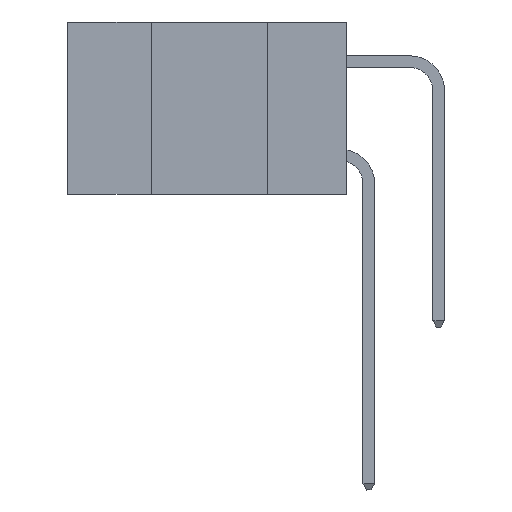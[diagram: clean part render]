
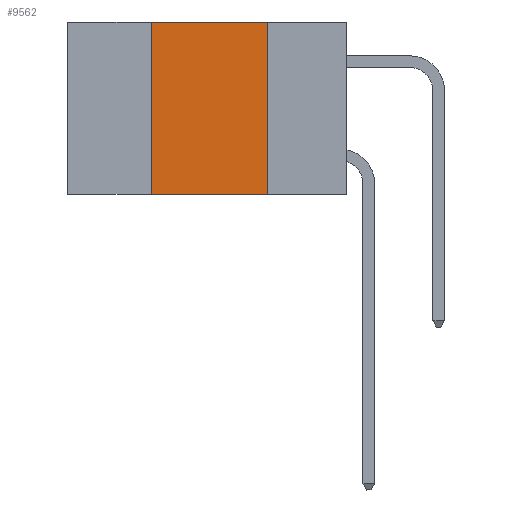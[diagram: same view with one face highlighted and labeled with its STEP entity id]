
A CAD part, left-side view. The second image highlights one B-rep face of the part: STEP entity #9562.
In plain terms, the highlighted planar face has unit normal (-1, 0, 0).
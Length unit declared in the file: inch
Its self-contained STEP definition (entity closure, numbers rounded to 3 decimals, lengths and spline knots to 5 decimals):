
#205 = DIRECTION ( 'NONE',  ( 0., -1., 0. ) ) ;
#664 = DIRECTION ( 'NONE',  ( 0., -1., 0. ) ) ;
#1040 = EDGE_CURVE ( 'NONE', #8376, #10038, #11381, .T. ) ;
#1263 = CARTESIAN_POINT ( 'NONE',  ( 0., 0.42, -0.37 ) ) ;
#1429 = ORIENTED_EDGE ( 'NONE', *, *, #1040, .F. ) ;
#1773 = LINE ( 'NONE', #12435, #2901 ) ;
#1972 = CARTESIAN_POINT ( 'NONE',  ( 0., 0.42, 0. ) ) ;
#2851 = CARTESIAN_POINT ( 'NONE',  ( 0., 0.6, 0. ) ) ;
#2901 = VECTOR ( 'NONE', #664, 39.37008 ) ;
#3010 = ORIENTED_EDGE ( 'NONE', *, *, #9655, .F. ) ;
#3097 = LINE ( 'NONE', #1972, #10056 ) ;
#3177 = DIRECTION ( 'NONE',  ( 0., 0., 1. ) ) ;
#3874 = EDGE_LOOP ( 'NONE', ( #1429, #3010, #5778, #11550 ) ) ;
#3967 = FACE_OUTER_BOUND ( 'NONE', #3874, .T. ) ;
#4256 = VERTEX_POINT ( 'NONE', #1263 ) ;
#4943 = CARTESIAN_POINT ( 'NONE',  ( 0., 0.17, 0. ) ) ;
#5388 = AXIS2_PLACEMENT_3D ( 'NONE', #2851, #13173, #6551 ) ;
#5728 = CARTESIAN_POINT ( 'NONE',  ( 0., 0.17, -0.37 ) ) ;
#5778 = ORIENTED_EDGE ( 'NONE', *, *, #14907, .F. ) ;
#6551 = DIRECTION ( 'NONE',  ( 0., 0., -1. ) ) ;
#7616 = EDGE_CURVE ( 'NONE', #4256, #10038, #1773, .T. ) ;
#8175 = CARTESIAN_POINT ( 'NONE',  ( 0., 0.17, 0. ) ) ;
#8376 = VERTEX_POINT ( 'NONE', #8175 ) ;
#9325 = VECTOR ( 'NONE', #15179, 39.37008 ) ;
#9562 = ADVANCED_FACE ( 'NONE', ( #3967 ), #11881, .F. ) ;
#9655 = EDGE_CURVE ( 'NONE', #13184, #8376, #16003, .T. ) ;
#10038 = VERTEX_POINT ( 'NONE', #5728 ) ;
#10056 = VECTOR ( 'NONE', #3177, 39.37008 ) ;
#10760 = CARTESIAN_POINT ( 'NONE',  ( 0., 0.6, 0. ) ) ;
#11381 = LINE ( 'NONE', #4943, #9325 ) ;
#11550 = ORIENTED_EDGE ( 'NONE', *, *, #7616, .T. ) ;
#11881 = PLANE ( 'NONE',  #5388 ) ;
#12435 = CARTESIAN_POINT ( 'NONE',  ( 0., 0.6, -0.37 ) ) ;
#12832 = CARTESIAN_POINT ( 'NONE',  ( 0., 0.42, 0. ) ) ;
#13173 = DIRECTION ( 'NONE',  ( 1., 0., 0. ) ) ;
#13184 = VERTEX_POINT ( 'NONE', #12832 ) ;
#14884 = VECTOR ( 'NONE', #205, 39.37008 ) ;
#14907 = EDGE_CURVE ( 'NONE', #4256, #13184, #3097, .T. ) ;
#15179 = DIRECTION ( 'NONE',  ( 0., 0., -1. ) ) ;
#16003 = LINE ( 'NONE', #10760, #14884 ) ;
